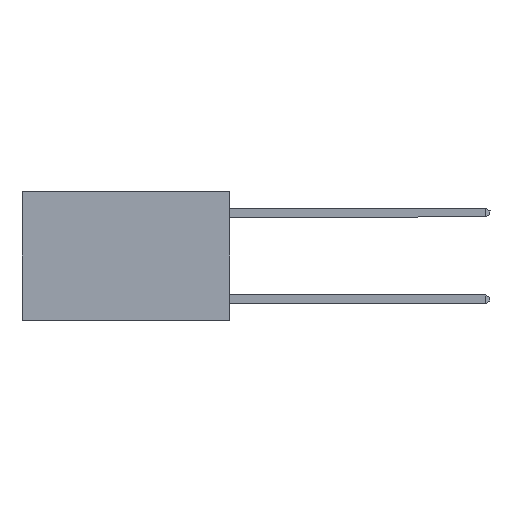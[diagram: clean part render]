
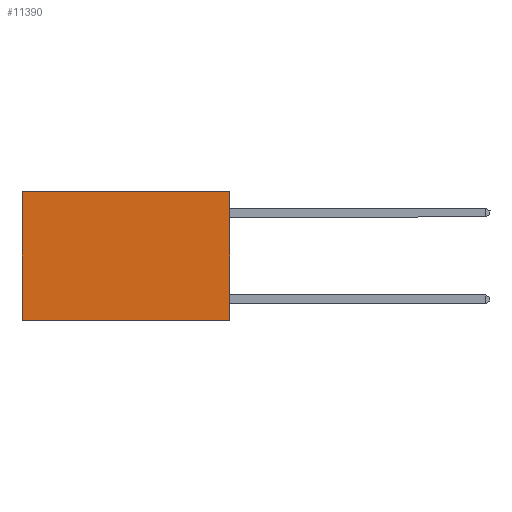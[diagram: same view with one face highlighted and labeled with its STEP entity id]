
A CAD part, left-side view. The second image highlights one B-rep face of the part: STEP entity #11390.
In plain terms, the highlighted planar face has unit normal (-1, 0, 0).
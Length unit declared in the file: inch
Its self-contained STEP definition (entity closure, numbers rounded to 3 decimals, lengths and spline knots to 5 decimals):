
#178 = ORIENTED_EDGE ( 'NONE', *, *, #574, .T. ) ;
#361 = CARTESIAN_POINT ( 'NONE',  ( 0.2625, 0., 0. ) ) ;
#398 = EDGE_CURVE ( 'NONE', #5645, #8113, #846, .T. ) ;
#574 = EDGE_CURVE ( 'NONE', #8113, #8101, #9819, .T. ) ;
#591 = EDGE_CURVE ( 'NONE', #4902, #8101, #2454, .T. ) ;
#651 = DIRECTION ( 'NONE',  ( 0., 0., -1. ) ) ;
#846 = LINE ( 'NONE', #11740, #5772 ) ;
#1110 = CARTESIAN_POINT ( 'NONE',  ( 0.2625, 0.6, -0.37 ) ) ;
#1405 = DIRECTION ( 'NONE',  ( 0., 0., -1. ) ) ;
#1550 = ORIENTED_EDGE ( 'NONE', *, *, #591, .F. ) ;
#1688 = DIRECTION ( 'NONE',  ( 0., 0., -1. ) ) ;
#2134 = CARTESIAN_POINT ( 'NONE',  ( 0.2625, 0., -0.37 ) ) ;
#2140 = CARTESIAN_POINT ( 'NONE',  ( 0.2625, 0.6, 0. ) ) ;
#2230 = FACE_OUTER_BOUND ( 'NONE', #11349, .T. ) ;
#2454 = LINE ( 'NONE', #4853, #11910 ) ;
#2730 = CARTESIAN_POINT ( 'NONE',  ( 0.2625, 0., 0. ) ) ;
#3578 = AXIS2_PLACEMENT_3D ( 'NONE', #361, #7163, #1405 ) ;
#4611 = LINE ( 'NONE', #2730, #7004 ) ;
#4707 = DIRECTION ( 'NONE',  ( 0., 1., 0. ) ) ;
#4853 = CARTESIAN_POINT ( 'NONE',  ( 0.2625, 0., -0.37 ) ) ;
#4902 = VERTEX_POINT ( 'NONE', #2134 ) ;
#5336 = PLANE ( 'NONE',  #3578 ) ;
#5638 = ORIENTED_EDGE ( 'NONE', *, *, #398, .T. ) ;
#5645 = VERTEX_POINT ( 'NONE', #10284 ) ;
#5772 = VECTOR ( 'NONE', #9045, 39.37008 ) ;
#6888 = CARTESIAN_POINT ( 'NONE',  ( 0.2625, 0.6, 0. ) ) ;
#7004 = VECTOR ( 'NONE', #1688, 39.37008 ) ;
#7163 = DIRECTION ( 'NONE',  ( 1., 0., 0. ) ) ;
#7474 = VECTOR ( 'NONE', #651, 39.37008 ) ;
#8101 = VERTEX_POINT ( 'NONE', #1110 ) ;
#8113 = VERTEX_POINT ( 'NONE', #6888 ) ;
#9045 = DIRECTION ( 'NONE',  ( 0., 1., 0. ) ) ;
#9122 = ORIENTED_EDGE ( 'NONE', *, *, #10701, .F. ) ;
#9819 = LINE ( 'NONE', #2140, #7474 ) ;
#10284 = CARTESIAN_POINT ( 'NONE',  ( 0.2625, 0., 0. ) ) ;
#10701 = EDGE_CURVE ( 'NONE', #5645, #4902, #4611, .T. ) ;
#11349 = EDGE_LOOP ( 'NONE', ( #178, #1550, #9122, #5638 ) ) ;
#11390 = ADVANCED_FACE ( 'NONE', ( #2230 ), #5336, .F. ) ;
#11740 = CARTESIAN_POINT ( 'NONE',  ( 0.2625, 0., 0. ) ) ;
#11910 = VECTOR ( 'NONE', #4707, 39.37008 ) ;
